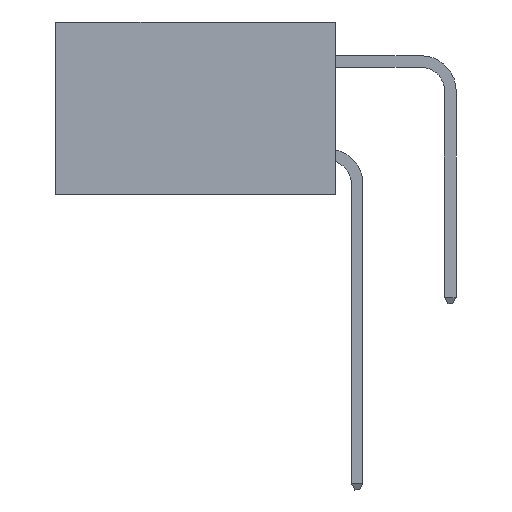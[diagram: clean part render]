
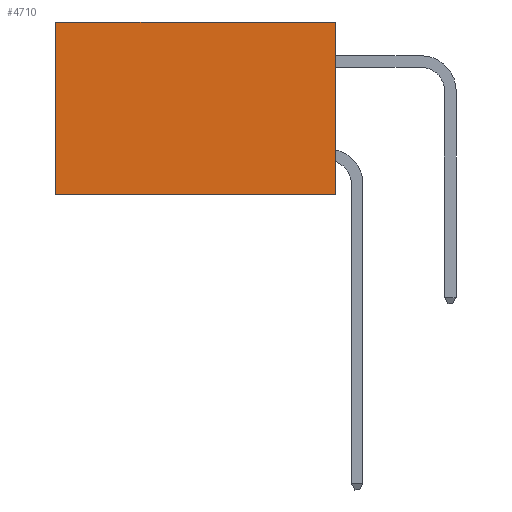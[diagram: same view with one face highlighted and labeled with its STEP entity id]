
A CAD part, left-side view. The second image highlights one B-rep face of the part: STEP entity #4710.
In plain terms, the highlighted planar face has unit normal (-1, 0, 0).
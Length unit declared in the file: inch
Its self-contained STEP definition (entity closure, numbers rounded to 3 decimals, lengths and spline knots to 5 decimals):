
#1661 = VECTOR ( 'NONE', #23787, 39.37008 ) ;
#2642 = ORIENTED_EDGE ( 'NONE', *, *, #12954, .F. ) ;
#2760 = DIRECTION ( 'NONE',  ( 0., 0., -1. ) ) ;
#3205 = ORIENTED_EDGE ( 'NONE', *, *, #8954, .T. ) ;
#4710 = ADVANCED_FACE ( 'NONE', ( #24539 ), #13482, .F. ) ;
#4808 = CARTESIAN_POINT ( 'NONE',  ( 0.2875, 0.6, 0. ) ) ;
#5109 = CARTESIAN_POINT ( 'NONE',  ( 0.2875, 0.6, 0. ) ) ;
#8855 = CARTESIAN_POINT ( 'NONE',  ( 0.2875, 0., 0. ) ) ;
#8954 = EDGE_CURVE ( 'NONE', #21922, #24534, #17273, .T. ) ;
#9628 = CARTESIAN_POINT ( 'NONE',  ( 0.2875, 0., 0. ) ) ;
#10695 = LINE ( 'NONE', #9628, #24467 ) ;
#10705 = ORIENTED_EDGE ( 'NONE', *, *, #25639, .T. ) ;
#11315 = VECTOR ( 'NONE', #2760, 39.37008 ) ;
#12954 = EDGE_CURVE ( 'NONE', #21922, #15721, #10695, .T. ) ;
#13482 = PLANE ( 'NONE',  #18954 ) ;
#13573 = DIRECTION ( 'NONE',  ( 0., 0., -1. ) ) ;
#14944 = CARTESIAN_POINT ( 'NONE',  ( 0.2875, 0., 0. ) ) ;
#15077 = CARTESIAN_POINT ( 'NONE',  ( 0.2875, 0.6, -0.37 ) ) ;
#15309 = DIRECTION ( 'NONE',  ( 1., 0., 0. ) ) ;
#15721 = VERTEX_POINT ( 'NONE', #23893 ) ;
#15761 = CARTESIAN_POINT ( 'NONE',  ( 0.2875, 0., -0.37 ) ) ;
#16027 = VECTOR ( 'NONE', #22807, 39.37008 ) ;
#16063 = LINE ( 'NONE', #15761, #1661 ) ;
#17273 = LINE ( 'NONE', #8855, #16027 ) ;
#18954 = AXIS2_PLACEMENT_3D ( 'NONE', #25059, #15309, #19110 ) ;
#19110 = DIRECTION ( 'NONE',  ( 0., 0., -1. ) ) ;
#19546 = EDGE_LOOP ( 'NONE', ( #10705, #25141, #2642, #3205 ) ) ;
#20003 = VERTEX_POINT ( 'NONE', #15077 ) ;
#21151 = EDGE_CURVE ( 'NONE', #15721, #20003, #16063, .T. ) ;
#21922 = VERTEX_POINT ( 'NONE', #14944 ) ;
#22807 = DIRECTION ( 'NONE',  ( 0., 1., 0. ) ) ;
#23787 = DIRECTION ( 'NONE',  ( 0., 1., 0. ) ) ;
#23893 = CARTESIAN_POINT ( 'NONE',  ( 0.2875, 0., -0.37 ) ) ;
#24467 = VECTOR ( 'NONE', #13573, 39.37008 ) ;
#24534 = VERTEX_POINT ( 'NONE', #5109 ) ;
#24539 = FACE_OUTER_BOUND ( 'NONE', #19546, .T. ) ;
#25059 = CARTESIAN_POINT ( 'NONE',  ( 0.2875, 0., 0. ) ) ;
#25141 = ORIENTED_EDGE ( 'NONE', *, *, #21151, .F. ) ;
#25639 = EDGE_CURVE ( 'NONE', #24534, #20003, #25645, .T. ) ;
#25645 = LINE ( 'NONE', #4808, #11315 ) ;
